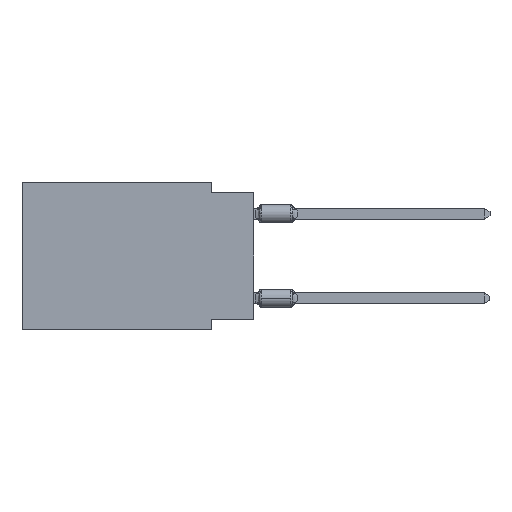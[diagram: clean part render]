
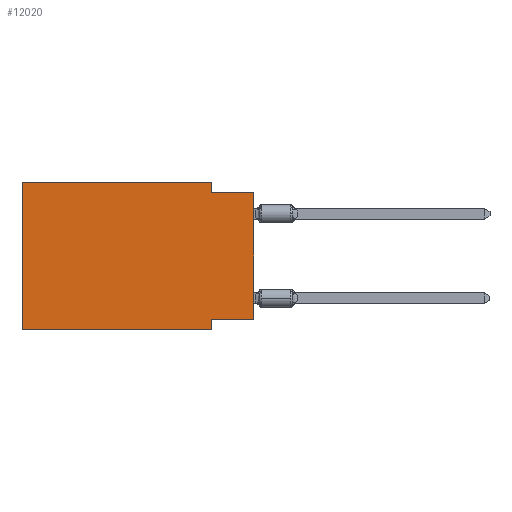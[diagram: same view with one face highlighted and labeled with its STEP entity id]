
A CAD part, left-side view. The second image highlights one B-rep face of the part: STEP entity #12020.
In plain terms, the highlighted planar face has unit normal (-1, 0, 0).
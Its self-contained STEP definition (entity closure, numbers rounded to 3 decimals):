
#510 = VERTEX_POINT ( 'NONE', #9972 ) ;
#617 = LINE ( 'NONE', #25405, #2807 ) ;
#715 = DIRECTION ( 'NONE',  ( 0., 1., 0. ) ) ;
#936 = CARTESIAN_POINT ( 'NONE',  ( 0., 13.97, 0. ) ) ;
#1455 = EDGE_LOOP ( 'NONE', ( #13888, #16947, #1646, #18424, #4987, #2223, #11890, #2270 ) ) ;
#1477 = VERTEX_POINT ( 'NONE', #12459 ) ;
#1646 = ORIENTED_EDGE ( 'NONE', *, *, #12572, .F. ) ;
#1832 = CARTESIAN_POINT ( 'NONE',  ( 0., 2.54, -8.89 ) ) ;
#2223 = ORIENTED_EDGE ( 'NONE', *, *, #14761, .T. ) ;
#2270 = ORIENTED_EDGE ( 'NONE', *, *, #27846, .F. ) ;
#2429 = DIRECTION ( 'NONE',  ( 0., -1., 0. ) ) ;
#2747 = LINE ( 'NONE', #7128, #21251 ) ;
#2807 = VECTOR ( 'NONE', #12759, 1000. ) ;
#2817 = CARTESIAN_POINT ( 'NONE',  ( 0., 13.97, -8.89 ) ) ;
#2928 = VECTOR ( 'NONE', #31013, 1000. ) ;
#3359 = DIRECTION ( 'NONE',  ( 1., 0., 0. ) ) ;
#4987 = ORIENTED_EDGE ( 'NONE', *, *, #29665, .F. ) ;
#5245 = LINE ( 'NONE', #2817, #9687 ) ;
#5728 = LINE ( 'NONE', #20169, #7656 ) ;
#6061 = LINE ( 'NONE', #18222, #2928 ) ;
#6765 = DIRECTION ( 'NONE',  ( 0., 0., -1. ) ) ;
#7128 = CARTESIAN_POINT ( 'NONE',  ( 0., 0., -0.635 ) ) ;
#7303 = VERTEX_POINT ( 'NONE', #14657 ) ;
#7656 = VECTOR ( 'NONE', #715, 1000. ) ;
#9211 = CARTESIAN_POINT ( 'NONE',  ( 0., 2.54, -8.89 ) ) ;
#9687 = VECTOR ( 'NONE', #12695, 1000. ) ;
#9845 = EDGE_CURVE ( 'NONE', #24190, #11332, #617, .T. ) ;
#9972 = CARTESIAN_POINT ( 'NONE',  ( 0., 2.54, -8.255 ) ) ;
#11194 = LINE ( 'NONE', #18155, #15676 ) ;
#11332 = VERTEX_POINT ( 'NONE', #28578 ) ;
#11727 = AXIS2_PLACEMENT_3D ( 'NONE', #936, #3359, #30567 ) ;
#11890 = ORIENTED_EDGE ( 'NONE', *, *, #15314, .F. ) ;
#11913 = CARTESIAN_POINT ( 'NONE',  ( 0., 13.97, 0. ) ) ;
#12020 = ADVANCED_FACE ( 'NONE', ( #12753 ), #30096, .F. ) ;
#12459 = CARTESIAN_POINT ( 'NONE',  ( 0., 0., -8.255 ) ) ;
#12572 = EDGE_CURVE ( 'NONE', #11332, #7303, #6061, .T. ) ;
#12695 = DIRECTION ( 'NONE',  ( 0., -1., 0. ) ) ;
#12753 = FACE_OUTER_BOUND ( 'NONE', #1455, .T. ) ;
#12759 = DIRECTION ( 'NONE',  ( 0., -1., 0. ) ) ;
#13308 = VECTOR ( 'NONE', #6765, 1000. ) ;
#13888 = ORIENTED_EDGE ( 'NONE', *, *, #23124, .T. ) ;
#14657 = CARTESIAN_POINT ( 'NONE',  ( 0., 2.54, -0.635 ) ) ;
#14761 = EDGE_CURVE ( 'NONE', #31208, #30505, #5245, .T. ) ;
#15314 = EDGE_CURVE ( 'NONE', #510, #30505, #26232, .T. ) ;
#15676 = VECTOR ( 'NONE', #30469, 1000. ) ;
#16947 = ORIENTED_EDGE ( 'NONE', *, *, #19985, .F. ) ;
#17814 = VECTOR ( 'NONE', #19307, 1000. ) ;
#18155 = CARTESIAN_POINT ( 'NONE',  ( 0., 0., 0. ) ) ;
#18222 = CARTESIAN_POINT ( 'NONE',  ( 0., 2.54, 0. ) ) ;
#18424 = ORIENTED_EDGE ( 'NONE', *, *, #9845, .F. ) ;
#18623 = CARTESIAN_POINT ( 'NONE',  ( 0., 13.97, -8.89 ) ) ;
#19307 = DIRECTION ( 'NONE',  ( 0., 0., 1. ) ) ;
#19472 = LINE ( 'NONE', #19638, #17814 ) ;
#19638 = CARTESIAN_POINT ( 'NONE',  ( 0., 13.97, 0. ) ) ;
#19985 = EDGE_CURVE ( 'NONE', #7303, #21114, #2747, .T. ) ;
#20169 = CARTESIAN_POINT ( 'NONE',  ( 0., 0., -8.255 ) ) ;
#21114 = VERTEX_POINT ( 'NONE', #31961 ) ;
#21251 = VECTOR ( 'NONE', #2429, 1000. ) ;
#23124 = EDGE_CURVE ( 'NONE', #1477, #21114, #11194, .T. ) ;
#24190 = VERTEX_POINT ( 'NONE', #11913 ) ;
#25405 = CARTESIAN_POINT ( 'NONE',  ( 0., 13.97, 0. ) ) ;
#26232 = LINE ( 'NONE', #9211, #13308 ) ;
#27846 = EDGE_CURVE ( 'NONE', #1477, #510, #5728, .T. ) ;
#28578 = CARTESIAN_POINT ( 'NONE',  ( 0., 2.54, 0. ) ) ;
#29665 = EDGE_CURVE ( 'NONE', #31208, #24190, #19472, .T. ) ;
#30096 = PLANE ( 'NONE',  #11727 ) ;
#30469 = DIRECTION ( 'NONE',  ( 0., 0., 1. ) ) ;
#30505 = VERTEX_POINT ( 'NONE', #1832 ) ;
#30567 = DIRECTION ( 'NONE',  ( 0., 0., -1. ) ) ;
#31013 = DIRECTION ( 'NONE',  ( 0., 0., -1. ) ) ;
#31208 = VERTEX_POINT ( 'NONE', #18623 ) ;
#31961 = CARTESIAN_POINT ( 'NONE',  ( 0., 0., -0.635 ) ) ;
